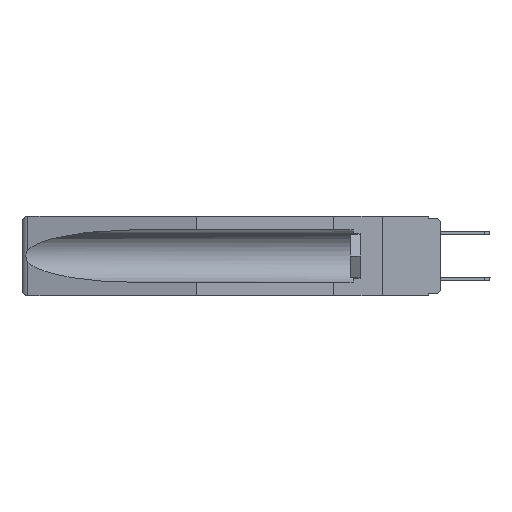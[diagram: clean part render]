
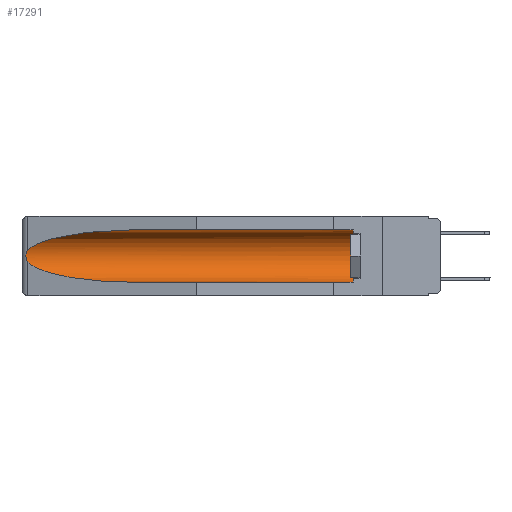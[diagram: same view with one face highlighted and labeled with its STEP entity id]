
A CAD part, left-side view. The second image highlights one B-rep face of the part: STEP entity #17291.
In plain terms, the highlighted cylindrical face has radius 2.857 mm (diameter 5.715 mm), a partial arc.
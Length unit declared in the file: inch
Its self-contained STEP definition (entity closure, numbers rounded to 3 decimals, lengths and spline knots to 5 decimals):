
#655 = CARTESIAN_POINT ( 'NONE',  ( 0.155, -0.30754, -0.059 ) ) ;
#1171 = CARTESIAN_POINT ( 'NONE',  ( 0.26537, 1.52718, -0.14972 ) ) ;
#1221 = CARTESIAN_POINT ( 'NONE',  ( 0.155, 0.126, -0.1715 ) ) ;
#1462 = DIRECTION ( 'NONE',  ( 0., -1., 0. ) ) ;
#1524 = ORIENTED_EDGE ( 'NONE', *, *, #13528, .T. ) ;
#1788 = FACE_OUTER_BOUND ( 'NONE', #18086, .T. ) ;
#1985 = DIRECTION ( 'NONE',  ( 0., 0., 1. ) ) ;
#2740 = VERTEX_POINT ( 'NONE', #21202 ) ;
#2921 = CARTESIAN_POINT ( 'NONE',  ( 0.2675, 1.53308, -0.16763 ) ) ;
#4568 = CARTESIAN_POINT ( 'NONE',  ( 0.155, 1.07973, -0.059 ) ) ;
#4614 = CARTESIAN_POINT ( 'NONE',  ( 0.21114, 1.30732, -0.059 ) ) ;
#4872 = CARTESIAN_POINT ( 'NONE',  ( 0.26655, 1.53094, -0.18657 ) ) ;
#5313 = EDGE_CURVE ( 'NONE', #23959, #10024, #8887, .T. ) ;
#5466 = CARTESIAN_POINT ( 'NONE',  ( 0.2673, 1.5327, -0.16383 ) ) ;
#6372 = CYLINDRICAL_SURFACE ( 'NONE', #22895, 0.1125 ) ;
#7073 = ORIENTED_EDGE ( 'NONE', *, *, #9100, .F. ) ;
#7109 = DIRECTION ( 'NONE',  ( 0., 1., 0. ) ) ;
#8232 = VECTOR ( 'NONE', #7109, 39.37008 ) ;
#8336 = CARTESIAN_POINT ( 'NONE',  ( 0.21114, 1.30732, -0.284 ) ) ;
#8887 = B_SPLINE_CURVE_WITH_KNOTS ( 'NONE', 3,
 ( #14992, #13049, #17063, #5466, #2921, #22826, #16547, #4872, #16985, #13215 ),
 .UNSPECIFIED., .F., .F.,
 ( 4, 2, 2, 2, 4 ),
 ( 0., 0.00029, 0.00058, 0.00087, 0.00117 ),
 .UNSPECIFIED. ) ;
#8931 = DIRECTION ( 'NONE',  ( 0., 1., 0. ) ) ;
#9021 = CARTESIAN_POINT ( 'NONE',  ( 0.155, 1.07973, -0.059 ) ) ;
#9100 = EDGE_CURVE ( 'NONE', #23884, #21064, #11897, .T. ) ;
#9596 = ORIENTED_EDGE ( 'NONE', *, *, #24648, .T. ) ;
#9599 = DIRECTION ( 'NONE',  ( 0., 1., 0. ) ) ;
#10024 = VERTEX_POINT ( 'NONE', #21959 ) ;
#10105 = CIRCLE ( 'NONE', #24999, 0.1125 ) ;
#10157 = CARTESIAN_POINT ( 'NONE',  ( 0.26537, 1.52718, -0.14972 ) ) ;
#10636 = EDGE_CURVE ( 'NONE', #23881, #23959, #20915, .T. ) ;
#11897 = LINE ( 'NONE', #12878, #8232 ) ;
#12878 = CARTESIAN_POINT ( 'NONE',  ( 0.155, -0.30754, -0.284 ) ) ;
#13049 = CARTESIAN_POINT ( 'NONE',  ( 0.26597, 1.52961, -0.15275 ) ) ;
#13215 = CARTESIAN_POINT ( 'NONE',  ( 0.26537, 1.52718, -0.19328 ) ) ;
#13528 = EDGE_CURVE ( 'NONE', #2740, #23881, #14481, .T. ) ;
#13530 = ORIENTED_EDGE ( 'NONE', *, *, #16107, .T. ) ;
#14026 = CARTESIAN_POINT ( 'NONE',  ( 0.155, 1.07973, -0.284 ) ) ;
#14272 = ORIENTED_EDGE ( 'NONE', *, *, #10636, .T. ) ;
#14481 = LINE ( 'NONE', #655, #21771 ) ;
#14678 = CARTESIAN_POINT ( 'NONE',  ( 0.155, 1.07973, -0.284 ) ) ;
#14992 = CARTESIAN_POINT ( 'NONE',  ( 0.26537, 1.52718, -0.14972 ) ) ;
#15453 = CARTESIAN_POINT ( 'NONE',  ( 0.155, -0.30754, -0.1715 ) ) ;
#15935 = CARTESIAN_POINT ( 'NONE',  ( 0.25451, 1.48313, -0.09465 ) ) ;
#16107 = EDGE_CURVE ( 'NONE', #10024, #21064, #19799, .T. ) ;
#16176 = CARTESIAN_POINT ( 'NONE',  ( 0.26537, 1.52718, -0.19328 ) ) ;
#16547 = CARTESIAN_POINT ( 'NONE',  ( 0.2673, 1.53269, -0.17917 ) ) ;
#16985 = CARTESIAN_POINT ( 'NONE',  ( 0.26597, 1.5296, -0.19026 ) ) ;
#17063 = CARTESIAN_POINT ( 'NONE',  ( 0.26654, 1.53092, -0.15636 ) ) ;
#17291 = ADVANCED_FACE ( 'NONE', ( #1788 ), #6372, .F. ) ;
#18086 = EDGE_LOOP ( 'NONE', ( #14272, #18827, #13530, #7073, #9596, #1524 ) ) ;
#18778 = DIRECTION ( 'NONE',  ( 0., 0., 1. ) ) ;
#18827 = ORIENTED_EDGE ( 'NONE', *, *, #5313, .T. ) ;
#19799 =( BOUNDED_CURVE ( )  B_SPLINE_CURVE ( 3, ( #16176, #21941, #8336, #14026 ),
 .UNSPECIFIED., .F., .F. ) 
 B_SPLINE_CURVE_WITH_KNOTS ( ( 4, 4 ),
 ( 0.1948, 1.5708 ),
 .UNSPECIFIED. ) 
 CURVE ( )  GEOMETRIC_REPRESENTATION_ITEM ( )  RATIONAL_B_SPLINE_CURVE ( ( 1., 0.848, 0.848, 1. ) ) 
 REPRESENTATION_ITEM ( '' )  );
#20245 = CARTESIAN_POINT ( 'NONE',  ( 0.155, 0.126, -0.284 ) ) ;
#20915 =( BOUNDED_CURVE ( )  B_SPLINE_CURVE ( 3, ( #9021, #4614, #15935, #10157 ),
 .UNSPECIFIED., .F., .F. ) 
 B_SPLINE_CURVE_WITH_KNOTS ( ( 4, 4 ),
 ( 4.71239, 6.08839 ),
 .UNSPECIFIED. ) 
 CURVE ( )  GEOMETRIC_REPRESENTATION_ITEM ( )  RATIONAL_B_SPLINE_CURVE ( ( 1., 0.848, 0.848, 1. ) ) 
 REPRESENTATION_ITEM ( '' )  );
#21064 = VERTEX_POINT ( 'NONE', #14678 ) ;
#21202 = CARTESIAN_POINT ( 'NONE',  ( 0.155, 0.126, -0.059 ) ) ;
#21771 = VECTOR ( 'NONE', #8931, 39.37008 ) ;
#21941 = CARTESIAN_POINT ( 'NONE',  ( 0.25451, 1.48313, -0.24835 ) ) ;
#21959 = CARTESIAN_POINT ( 'NONE',  ( 0.26537, 1.52718, -0.19328 ) ) ;
#22826 = CARTESIAN_POINT ( 'NONE',  ( 0.2675, 1.53308, -0.17534 ) ) ;
#22895 = AXIS2_PLACEMENT_3D ( 'NONE', #15453, #9599, #1985 ) ;
#23881 = VERTEX_POINT ( 'NONE', #4568 ) ;
#23884 = VERTEX_POINT ( 'NONE', #20245 ) ;
#23959 = VERTEX_POINT ( 'NONE', #1171 ) ;
#24648 = EDGE_CURVE ( 'NONE', #23884, #2740, #10105, .T. ) ;
#24999 = AXIS2_PLACEMENT_3D ( 'NONE', #1221, #1462, #18778 ) ;
